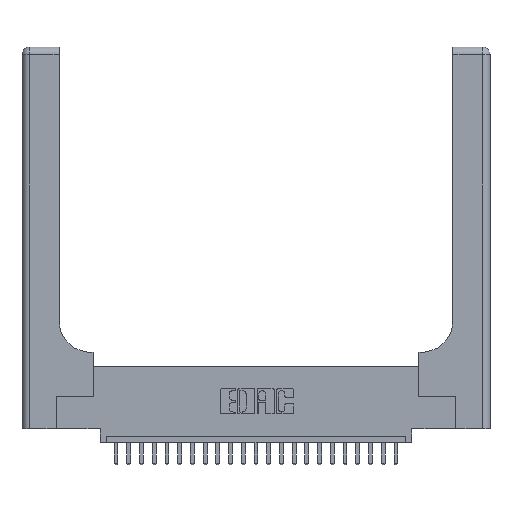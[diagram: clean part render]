
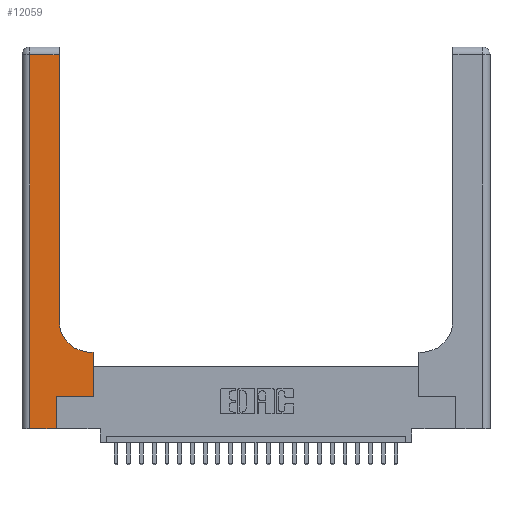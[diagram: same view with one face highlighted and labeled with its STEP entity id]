
A CAD part, top view. The second image highlights one B-rep face of the part: STEP entity #12059.
In plain terms, the highlighted planar face has unit normal (0, 0, 1).
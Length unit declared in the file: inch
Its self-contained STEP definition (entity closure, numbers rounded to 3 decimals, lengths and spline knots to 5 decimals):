
#684 = ORIENTED_EDGE ( 'NONE', *, *, #22017, .T. ) ;
#741 = CARTESIAN_POINT ( 'NONE',  ( 0., 3., 0.37 ) ) ;
#757 = ORIENTED_EDGE ( 'NONE', *, *, #19939, .T. ) ;
#988 = EDGE_LOOP ( 'NONE', ( #3182, #757, #3483, #10458, #24622, #684, #4033, #13695, #3812 ) ) ;
#1238 = LINE ( 'NONE', #16357, #24766 ) ;
#1332 = CARTESIAN_POINT ( 'NONE',  ( 0.269, 0., 0.37 ) ) ;
#1503 = EDGE_CURVE ( 'NONE', #16725, #24545, #10144, .T. ) ;
#1583 = CARTESIAN_POINT ( 'NONE',  ( 0.5415, 0.6, 0.37 ) ) ;
#2397 = EDGE_CURVE ( 'NONE', #24445, #7605, #1238, .T. ) ;
#2477 = VECTOR ( 'NONE', #9245, 39.37008 ) ;
#2486 = DIRECTION ( 'NONE',  ( 0., -1., 0. ) ) ;
#3182 = ORIENTED_EDGE ( 'NONE', *, *, #23898, .T. ) ;
#3203 = VERTEX_POINT ( 'NONE', #17694 ) ;
#3483 = ORIENTED_EDGE ( 'NONE', *, *, #15391, .T. ) ;
#3812 = ORIENTED_EDGE ( 'NONE', *, *, #14492, .T. ) ;
#3993 = CARTESIAN_POINT ( 'NONE',  ( 0.06, 0., 0.37 ) ) ;
#4033 = ORIENTED_EDGE ( 'NONE', *, *, #20624, .T. ) ;
#4039 = LINE ( 'NONE', #20019, #7981 ) ;
#4842 = CARTESIAN_POINT ( 'NONE',  ( 0.5415, 0.85, 0.37 ) ) ;
#4844 = LINE ( 'NONE', #5728, #18293 ) ;
#4877 = CARTESIAN_POINT ( 'NONE',  ( 0.269, 0.25, 0.37 ) ) ;
#5023 = CARTESIAN_POINT ( 'NONE',  ( 0.5585, 0.6, 0.37 ) ) ;
#5578 = CARTESIAN_POINT ( 'NONE',  ( 0.2915, 0.6, 0.37 ) ) ;
#5728 = CARTESIAN_POINT ( 'NONE',  ( 0., 2.94, 0.37 ) ) ;
#6481 = LINE ( 'NONE', #20109, #12550 ) ;
#6785 = LINE ( 'NONE', #19051, #13192 ) ;
#7226 = FACE_OUTER_BOUND ( 'NONE', #988, .T. ) ;
#7605 = VERTEX_POINT ( 'NONE', #13549 ) ;
#7981 = VECTOR ( 'NONE', #8285, 39.37008 ) ;
#8285 = DIRECTION ( 'NONE',  ( 1., 0., 0. ) ) ;
#8568 = DIRECTION ( 'NONE',  ( 0., 1., 0. ) ) ;
#8698 = DIRECTION ( 'NONE',  ( 1., 0., 0. ) ) ;
#9245 = DIRECTION ( 'NONE',  ( -1., 0., 0. ) ) ;
#10144 = LINE ( 'NONE', #5578, #2477 ) ;
#10458 = ORIENTED_EDGE ( 'NONE', *, *, #24765, .T. ) ;
#11469 = VERTEX_POINT ( 'NONE', #16679 ) ;
#12059 = ADVANCED_FACE ( 'NONE', ( #7226 ), #12427, .F. ) ;
#12427 = PLANE ( 'NONE',  #17764 ) ;
#12550 = VECTOR ( 'NONE', #2486, 39.37008 ) ;
#12671 = DIRECTION ( 'NONE',  ( 1., 0., 0. ) ) ;
#13192 = VECTOR ( 'NONE', #15167, 39.37008 ) ;
#13390 = DIRECTION ( 'NONE',  ( 0., 1., 0. ) ) ;
#13549 = CARTESIAN_POINT ( 'NONE',  ( 0.269, 0.25, 0.37 ) ) ;
#13695 = ORIENTED_EDGE ( 'NONE', *, *, #1503, .T. ) ;
#14023 = VERTEX_POINT ( 'NONE', #22675 ) ;
#14267 = VERTEX_POINT ( 'NONE', #3993 ) ;
#14305 = VERTEX_POINT ( 'NONE', #17825 ) ;
#14492 = EDGE_CURVE ( 'NONE', #24545, #3203, #14755, .T. ) ;
#14755 = CIRCLE ( 'NONE', #22674, 0.25 ) ;
#15167 = DIRECTION ( 'NONE',  ( 0., 1., 0. ) ) ;
#15391 = EDGE_CURVE ( 'NONE', #14023, #14267, #6481, .T. ) ;
#16008 = VECTOR ( 'NONE', #8698, 39.37008 ) ;
#16357 = CARTESIAN_POINT ( 'NONE',  ( 0.269, 0., 0.37 ) ) ;
#16679 = CARTESIAN_POINT ( 'NONE',  ( 0.5585, 0.25, 0.37 ) ) ;
#16725 = VERTEX_POINT ( 'NONE', #5023 ) ;
#16749 = LINE ( 'NONE', #17444, #25283 ) ;
#17444 = CARTESIAN_POINT ( 'NONE',  ( 0.5585, 0.25, 0.37 ) ) ;
#17694 = CARTESIAN_POINT ( 'NONE',  ( 0.2915, 0.85, 0.37 ) ) ;
#17764 = AXIS2_PLACEMENT_3D ( 'NONE', #741, #24257, #22582 ) ;
#17825 = CARTESIAN_POINT ( 'NONE',  ( 0.2915, 2.94, 0.37 ) ) ;
#18293 = VECTOR ( 'NONE', #19418, 39.37008 ) ;
#18423 = DIRECTION ( 'NONE',  ( 0., 0., -1. ) ) ;
#19051 = CARTESIAN_POINT ( 'NONE',  ( 0.2915, 3., 0.37 ) ) ;
#19418 = DIRECTION ( 'NONE',  ( -1., 0., 0. ) ) ;
#19939 = EDGE_CURVE ( 'NONE', #14305, #14023, #4844, .T. ) ;
#20019 = CARTESIAN_POINT ( 'NONE',  ( 0., 0., 0.37 ) ) ;
#20109 = CARTESIAN_POINT ( 'NONE',  ( 0.06, 3., 0.37 ) ) ;
#20624 = EDGE_CURVE ( 'NONE', #11469, #16725, #16749, .T. ) ;
#21266 = LINE ( 'NONE', #4877, #16008 ) ;
#22017 = EDGE_CURVE ( 'NONE', #7605, #11469, #21266, .T. ) ;
#22582 = DIRECTION ( 'NONE',  ( -1., 0., 0. ) ) ;
#22675 = CARTESIAN_POINT ( 'NONE',  ( 0.06, 2.94, 0.37 ) ) ;
#22674 = AXIS2_PLACEMENT_3D ( 'NONE', #4842, #18423, #12671 ) ;
#23898 = EDGE_CURVE ( 'NONE', #3203, #14305, #6785, .T. ) ;
#24257 = DIRECTION ( 'NONE',  ( 0., 0., -1. ) ) ;
#24445 = VERTEX_POINT ( 'NONE', #1332 ) ;
#24545 = VERTEX_POINT ( 'NONE', #1583 ) ;
#24622 = ORIENTED_EDGE ( 'NONE', *, *, #2397, .T. ) ;
#24765 = EDGE_CURVE ( 'NONE', #14267, #24445, #4039, .T. ) ;
#24766 = VECTOR ( 'NONE', #8568, 39.37008 ) ;
#25283 = VECTOR ( 'NONE', #13390, 39.37008 ) ;
